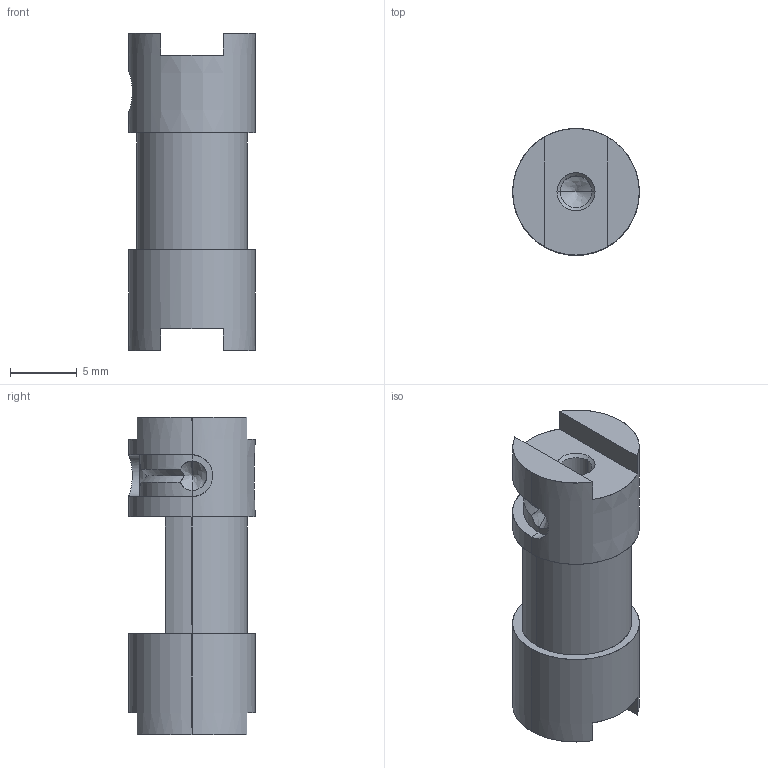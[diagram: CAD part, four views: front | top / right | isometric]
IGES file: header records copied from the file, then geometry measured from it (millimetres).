
Start section: SolidWorks IGES file using analytic representation for surfaces
Global section: file name: Selector.igs; native system: SolidWorks 2015; preprocessor: SolidWorks 2015; author: WarFairy; date: 150711.203116; units: millimetre
Bounding box: 9.46 x 9.46 x 23.71 mm (x, y, z)
Surface area: 982.5 mm2 (no closed solid volume)
Topology: 0 solids, 0 shells, 47 faces, 641 edges, 633 vertices
Faces by surface type: revolution 30, bspline 17
